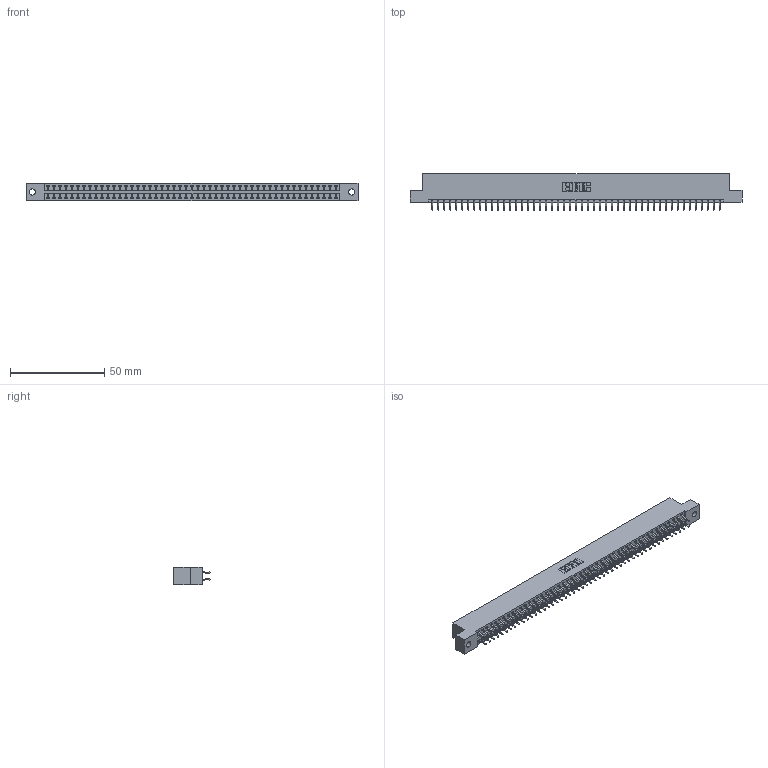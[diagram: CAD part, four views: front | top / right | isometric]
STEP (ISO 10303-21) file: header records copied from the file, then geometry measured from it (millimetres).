
FILE_DESCRIPTION (( 'STEP AP203' ), '1' );
FILE_NAME ('396-098-556-202.STEP', '2018-09-14T05:34:57', ( '' ), ( '' ), 'SwSTEP 2.0', 'SolidWorks 2016', '' );
FILE_SCHEMA (( 'CONFIG_CONTROL_DESIGN' ));
Length unit declared in the file: inch
Products named in the file (3): 346 Part_Flush Mounting Lugs - 0.128 Dia; 345-292-001_556 Tail; 396-098-556-202
Assembly tree (99 placements, depth 2):
  396-098-556-202
    346 Part_Flush Mounting Lugs - 0.128 Dia
    345-292-001_556 Tail  x98
Bounding box: 176.15 x 19.57 x 9.4 mm (x, y, z)
Volume: 17190.5 mm3; surface area: 23379.3 mm2
Topology: 99 solids, 99 shells, 5806 faces, 17283 edges, 11390 vertices
Faces by surface type: plane 3898, cylinder 1908
Entity records: 31259 total; most frequent: CARTESIAN_POINT 5156, ORIENTED_EDGE 5078, DIRECTION 4583, EDGE_CURVE 2539, VECTOR 2203, LINE 2203, VERTEX_POINT 1690, AXIS2_PLACEMENT_3D 1190
